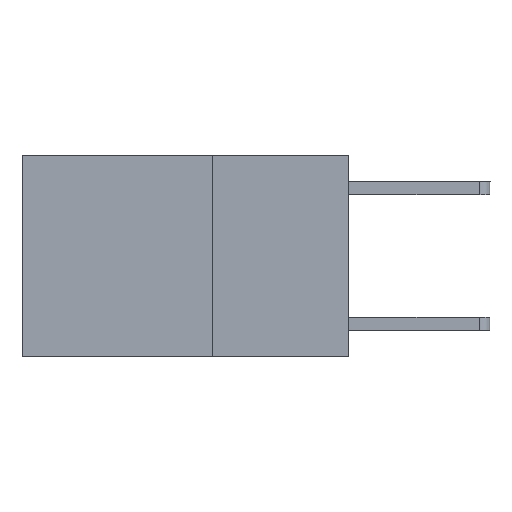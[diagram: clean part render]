
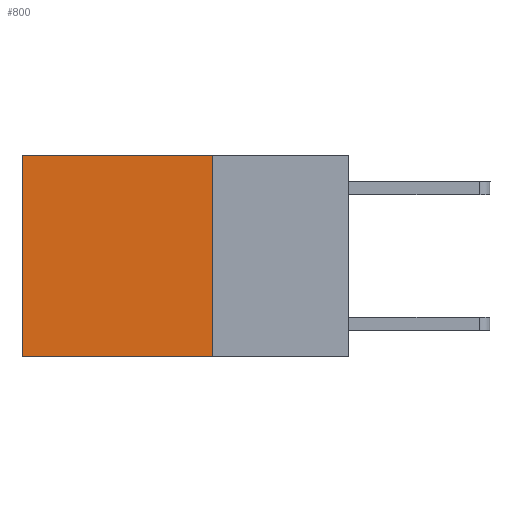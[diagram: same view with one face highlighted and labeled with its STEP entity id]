
A CAD part, left-side view. The second image highlights one B-rep face of the part: STEP entity #800.
In plain terms, the highlighted planar face has unit normal (-1, 0, 0).
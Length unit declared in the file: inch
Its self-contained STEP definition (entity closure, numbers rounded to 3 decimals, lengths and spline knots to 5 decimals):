
#3 = DIRECTION ( 'NONE',  ( 0., 0., -1. ) ) ;
#48 = ORIENTED_EDGE ( 'NONE', *, *, #7730, .F. ) ;
#61 = PLANE ( 'NONE',  #5569 ) ;
#564 = LINE ( 'NONE', #4618, #962 ) ;
#682 = DIRECTION ( 'NONE',  ( 1., 0., 0. ) ) ;
#701 = LINE ( 'NONE', #5890, #7845 ) ;
#773 = DIRECTION ( 'NONE',  ( 0., 0., -1. ) ) ;
#800 = ADVANCED_FACE ( 'NONE', ( #6000 ), #61, .F. ) ;
#946 = EDGE_CURVE ( 'NONE', #6543, #6560, #5640, .T. ) ;
#962 = VECTOR ( 'NONE', #773, 39.37008 ) ;
#2277 = CARTESIAN_POINT ( 'NONE',  ( 0.2625, 0.25, 0. ) ) ;
#2305 = DIRECTION ( 'NONE',  ( 0., 1., 0. ) ) ;
#2518 = EDGE_LOOP ( 'NONE', ( #5405, #3960, #48, #4140 ) ) ;
#3772 = VECTOR ( 'NONE', #5652, 39.37008 ) ;
#3960 = ORIENTED_EDGE ( 'NONE', *, *, #946, .F. ) ;
#4140 = ORIENTED_EDGE ( 'NONE', *, *, #6573, .T. ) ;
#4292 = CARTESIAN_POINT ( 'NONE',  ( 0.2625, 0.6, -0.37 ) ) ;
#4618 = CARTESIAN_POINT ( 'NONE',  ( 0.2625, 0.6, 0. ) ) ;
#5066 = EDGE_CURVE ( 'NONE', #7888, #6560, #564, .T. ) ;
#5193 = VECTOR ( 'NONE', #2305, 39.37008 ) ;
#5405 = ORIENTED_EDGE ( 'NONE', *, *, #5066, .T. ) ;
#5426 = CARTESIAN_POINT ( 'NONE',  ( 0.2625, 0.25, 0. ) ) ;
#5569 = AXIS2_PLACEMENT_3D ( 'NONE', #5426, #682, #8077 ) ;
#5640 = LINE ( 'NONE', #8300, #5193 ) ;
#5652 = DIRECTION ( 'NONE',  ( 0., 1., 0. ) ) ;
#5890 = CARTESIAN_POINT ( 'NONE',  ( 0.2625, 0.25, 0. ) ) ;
#6000 = FACE_OUTER_BOUND ( 'NONE', #2518, .T. ) ;
#6543 = VERTEX_POINT ( 'NONE', #8224 ) ;
#6560 = VERTEX_POINT ( 'NONE', #4292 ) ;
#6573 = EDGE_CURVE ( 'NONE', #8327, #7888, #7516, .T. ) ;
#6702 = CARTESIAN_POINT ( 'NONE',  ( 0.2625, 0.25, 0. ) ) ;
#7516 = LINE ( 'NONE', #2277, #3772 ) ;
#7719 = CARTESIAN_POINT ( 'NONE',  ( 0.2625, 0.6, 0. ) ) ;
#7730 = EDGE_CURVE ( 'NONE', #8327, #6543, #701, .T. ) ;
#7845 = VECTOR ( 'NONE', #3, 39.37008 ) ;
#7888 = VERTEX_POINT ( 'NONE', #7719 ) ;
#8077 = DIRECTION ( 'NONE',  ( 0., 0., -1. ) ) ;
#8224 = CARTESIAN_POINT ( 'NONE',  ( 0.2625, 0.25, -0.37 ) ) ;
#8300 = CARTESIAN_POINT ( 'NONE',  ( 0.2625, 0.25, -0.37 ) ) ;
#8327 = VERTEX_POINT ( 'NONE', #6702 ) ;
